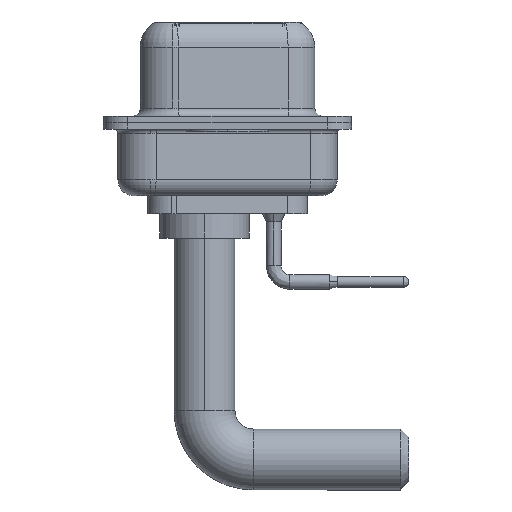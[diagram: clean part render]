
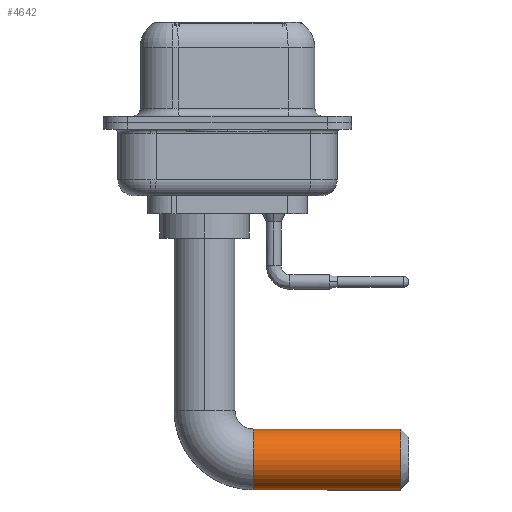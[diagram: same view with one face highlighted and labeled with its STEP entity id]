
A CAD part, left-side view. The second image highlights one B-rep face of the part: STEP entity #4642.
In plain terms, the highlighted cylindrical face has radius 1.875 mm (diameter 3.75 mm), a partial arc.
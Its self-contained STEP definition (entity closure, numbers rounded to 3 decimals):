
#1037 = DIRECTION ( 'NONE',  ( 0., -1., 0. ) ) ;
#1129 = CARTESIAN_POINT ( 'NONE',  ( 0., -3., -15.505 ) ) ;
#1676 = CIRCLE ( 'NONE', #1990, 1.875 ) ;
#1990 = AXIS2_PLACEMENT_3D ( 'NONE', #11429, #8268, #14098 ) ;
#2128 = CARTESIAN_POINT ( 'NONE',  ( 0., -12.07, -15.505 ) ) ;
#2269 = DIRECTION ( 'NONE',  ( 0., 0., -1. ) ) ;
#2875 = VECTOR ( 'NONE', #14725, 1000. ) ;
#4642 = ADVANCED_FACE ( 'NONE', ( #7089 ), #18866, .T. ) ;
#4905 = VERTEX_POINT ( 'NONE', #2128 ) ;
#5463 = VERTEX_POINT ( 'NONE', #14601 ) ;
#6167 = CARTESIAN_POINT ( 'NONE',  ( 0., -12.07, -11.755 ) ) ;
#6225 = ORIENTED_EDGE ( 'NONE', *, *, #13369, .T. ) ;
#6790 = DIRECTION ( 'NONE',  ( 0., -1., 0. ) ) ;
#6899 = DIRECTION ( 'NONE',  ( 0., 1., 0. ) ) ;
#7089 = FACE_OUTER_BOUND ( 'NONE', #11866, .T. ) ;
#7163 = ORIENTED_EDGE ( 'NONE', *, *, #9374, .F. ) ;
#7500 = VERTEX_POINT ( 'NONE', #12700 ) ;
#8268 = DIRECTION ( 'NONE',  ( 0., -1., 0. ) ) ;
#9374 = EDGE_CURVE ( 'NONE', #5463, #11731, #16493, .T. ) ;
#10658 = VECTOR ( 'NONE', #1037, 1000. ) ;
#10697 = ORIENTED_EDGE ( 'NONE', *, *, #10914, .T. ) ;
#10914 = EDGE_CURVE ( 'NONE', #4905, #11731, #18133, .T. ) ;
#11244 = AXIS2_PLACEMENT_3D ( 'NONE', #14111, #6899, #2269 ) ;
#11429 = CARTESIAN_POINT ( 'NONE',  ( 0., -3., -13.63 ) ) ;
#11731 = VERTEX_POINT ( 'NONE', #6167 ) ;
#11866 = EDGE_LOOP ( 'NONE', ( #7163, #13402, #6225, #10697 ) ) ;
#12700 = CARTESIAN_POINT ( 'NONE',  ( 0., -3., -15.505 ) ) ;
#13107 = AXIS2_PLACEMENT_3D ( 'NONE', #16233, #6790, #14481 ) ;
#13369 = EDGE_CURVE ( 'NONE', #7500, #4905, #17660, .T. ) ;
#13402 = ORIENTED_EDGE ( 'NONE', *, *, #18385, .T. ) ;
#14098 = DIRECTION ( 'NONE',  ( -1., 0., 0. ) ) ;
#14111 = CARTESIAN_POINT ( 'NONE',  ( 0., -12.07, -13.63 ) ) ;
#14481 = DIRECTION ( 'NONE',  ( 0., 0., -1. ) ) ;
#14601 = CARTESIAN_POINT ( 'NONE',  ( 0., -3., -11.755 ) ) ;
#14725 = DIRECTION ( 'NONE',  ( 0., -1., 0. ) ) ;
#14918 = CARTESIAN_POINT ( 'NONE',  ( 0., -3., -11.755 ) ) ;
#16233 = CARTESIAN_POINT ( 'NONE',  ( 0., -3., -13.63 ) ) ;
#16493 = LINE ( 'NONE', #14918, #2875 ) ;
#17660 = LINE ( 'NONE', #1129, #10658 ) ;
#18133 = CIRCLE ( 'NONE', #11244, 1.875 ) ;
#18385 = EDGE_CURVE ( 'NONE', #5463, #7500, #1676, .T. ) ;
#18866 = CYLINDRICAL_SURFACE ( 'NONE', #13107, 1.875 ) ;
